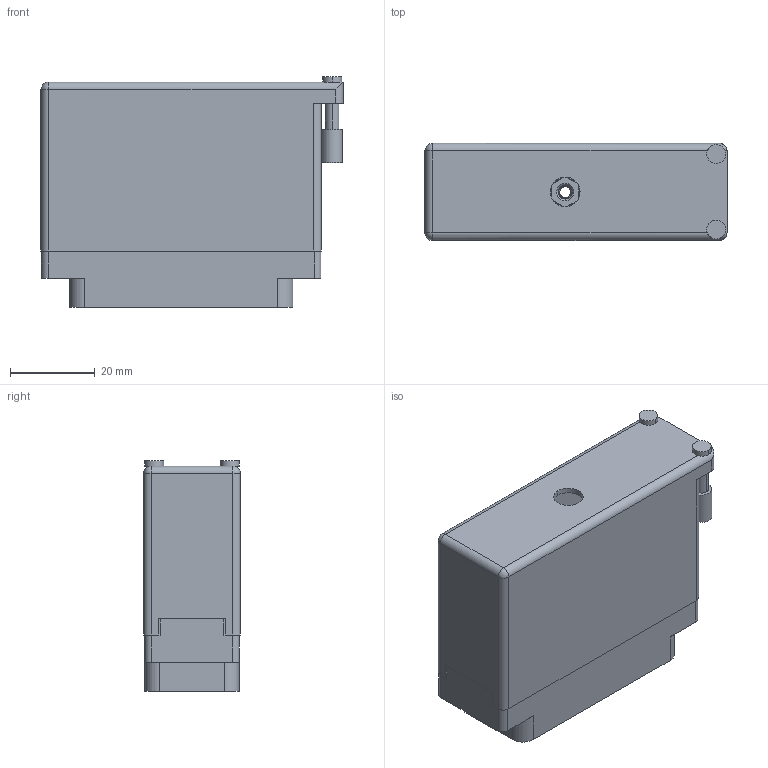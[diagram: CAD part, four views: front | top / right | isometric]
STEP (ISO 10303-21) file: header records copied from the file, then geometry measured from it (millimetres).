
FILE_DESCRIPTION (( 'STEP AP203' ), '1' );
FILE_NAME ('516-056-500-356.STEP', '2020-03-10T06:40:37', ( '' ), ( '' ), 'SwSTEP 2.0', 'SolidWorks 2016', '' );
FILE_SCHEMA (( 'CONFIG_CONTROL_DESIGN' ));
Length unit declared in the file: inch
Products named in the file (5): 516-292-001_500 Contact; 516 Plug Insulator_056; 516-056-500-356; 516-252-035-100_516-252-035-100; 516-230-001_Metal - 056 Side Entry
Assembly tree (59 placements, depth 2):
  516-056-500-356
    516 Plug Insulator_056
    516-292-001_500 Contact  x56
    516-230-001_Metal - 056 Side Entry
    516-252-035-100_516-252-035-100
Bounding box: 71.12 x 22.83 x 54.31 mm (x, y, z)
Volume: 24079.2 mm3; surface area: 42321.5 mm2
Topology: 59 solids, 59 shells, 5589 faces, 16221 edges, 10768 vertices
Faces by surface type: plane 3349, cylinder 1884, bspline 342, cone 12, sphere 2
Entity records: 51721 total; most frequent: CARTESIAN_POINT 11100, ORIENTED_EDGE 8238, DIRECTION 7947, EDGE_CURVE 4119, LINE 3031, VECTOR 3031, VERTEX_POINT 2738, AXIS2_PLACEMENT_3D 2458
